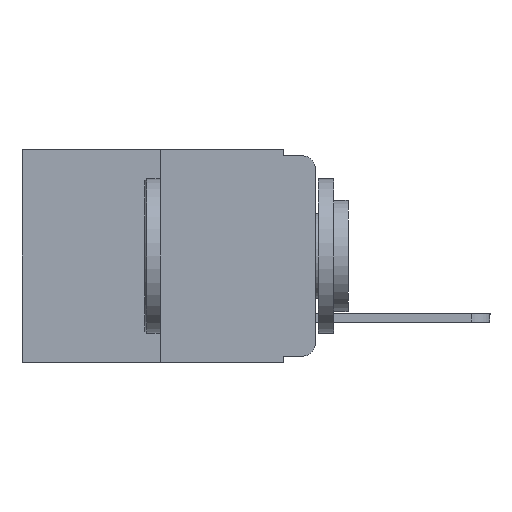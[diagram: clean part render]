
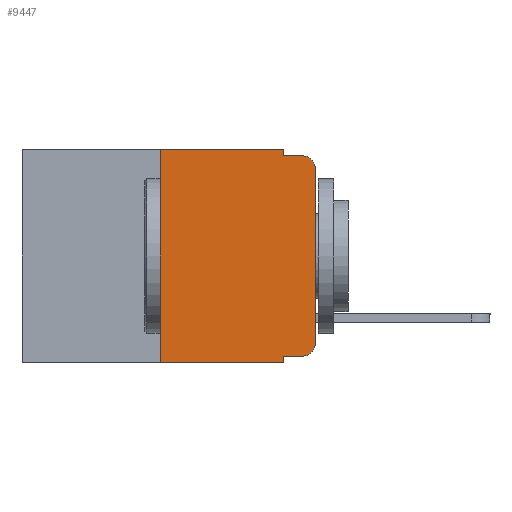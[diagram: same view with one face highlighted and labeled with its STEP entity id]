
A CAD part, left-side view. The second image highlights one B-rep face of the part: STEP entity #9447.
In plain terms, the highlighted planar face has unit normal (-1, 0, 0).
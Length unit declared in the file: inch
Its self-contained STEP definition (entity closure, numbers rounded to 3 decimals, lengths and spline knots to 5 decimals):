
#751 = EDGE_CURVE ( 'NONE', #3097, #4603, #8478, .T. ) ;
#780 = VERTEX_POINT ( 'NONE', #5957 ) ;
#983 = ORIENTED_EDGE ( 'NONE', *, *, #8936, .F. ) ;
#1001 = CARTESIAN_POINT ( 'NONE',  ( 0., 0.25, -0.343 ) ) ;
#1039 = VERTEX_POINT ( 'NONE', #2042 ) ;
#1045 = CARTESIAN_POINT ( 'NONE',  ( 0., 0.25, 0. ) ) ;
#1161 = LINE ( 'NONE', #1045, #6278 ) ;
#1274 = AXIS2_PLACEMENT_3D ( 'NONE', #11518, #5356, #2969 ) ;
#1533 = VECTOR ( 'NONE', #5927, 39.37008 ) ;
#1597 = CARTESIAN_POINT ( 'NONE',  ( 0., 0.051, 0. ) ) ;
#1614 = CARTESIAN_POINT ( 'NONE',  ( 0., 0.473, 0. ) ) ;
#1689 = ORIENTED_EDGE ( 'NONE', *, *, #6660, .F. ) ;
#1763 = CARTESIAN_POINT ( 'NONE',  ( 0., 0.02, -0.333 ) ) ;
#1821 = LINE ( 'NONE', #11740, #11657 ) ;
#1855 = LINE ( 'NONE', #9498, #1533 ) ;
#2042 = CARTESIAN_POINT ( 'NONE',  ( 0., 0.051, 0. ) ) ;
#2154 = CARTESIAN_POINT ( 'NONE',  ( 0., 0., 0. ) ) ;
#2172 = EDGE_CURVE ( 'NONE', #10506, #4603, #2993, .T. ) ;
#2265 = DIRECTION ( 'NONE',  ( 0., 0., 1. ) ) ;
#2562 = DIRECTION ( 'NONE',  ( 0., -1., 0. ) ) ;
#2915 = VECTOR ( 'NONE', #6635, 39.37008 ) ;
#2969 = DIRECTION ( 'NONE',  ( 0., 0., -1. ) ) ;
#2993 = CIRCLE ( 'NONE', #1274, 0.02 ) ;
#3045 = CARTESIAN_POINT ( 'NONE',  ( 0., 0.051, -0.01 ) ) ;
#3097 = VERTEX_POINT ( 'NONE', #11881 ) ;
#3306 = LINE ( 'NONE', #1597, #5958 ) ;
#3740 = CARTESIAN_POINT ( 'NONE',  ( 0., 0.02, -0.01 ) ) ;
#3771 = DIRECTION ( 'NONE',  ( 0., 0., -1. ) ) ;
#3786 = ORIENTED_EDGE ( 'NONE', *, *, #2172, .T. ) ;
#4203 = DIRECTION ( 'NONE',  ( 0., 0., 1. ) ) ;
#4301 = EDGE_CURVE ( 'NONE', #4403, #10506, #10620, .T. ) ;
#4403 = VERTEX_POINT ( 'NONE', #8969 ) ;
#4542 = CARTESIAN_POINT ( 'NONE',  ( 0., 0.051, -0.333 ) ) ;
#4603 = VERTEX_POINT ( 'NONE', #3740 ) ;
#5356 = DIRECTION ( 'NONE',  ( -1., 0., 0. ) ) ;
#5506 = DIRECTION ( 'NONE',  ( 0., -1., 0. ) ) ;
#5724 = PLANE ( 'NONE',  #7499 ) ;
#5766 = VECTOR ( 'NONE', #2265, 39.37008 ) ;
#5791 = ORIENTED_EDGE ( 'NONE', *, *, #4301, .T. ) ;
#5832 = EDGE_CURVE ( 'NONE', #9545, #4403, #11825, .T. ) ;
#5927 = DIRECTION ( 'NONE',  ( 0., -1., 0. ) ) ;
#5936 = EDGE_CURVE ( 'NONE', #10446, #780, #6472, .T. ) ;
#5957 = CARTESIAN_POINT ( 'NONE',  ( 0., 0.051, -0.343 ) ) ;
#5958 = VECTOR ( 'NONE', #7617, 39.37008 ) ;
#6278 = VECTOR ( 'NONE', #4203, 39.37008 ) ;
#6288 = CARTESIAN_POINT ( 'NONE',  ( 0., 0., -0.03 ) ) ;
#6472 = LINE ( 'NONE', #9164, #2915 ) ;
#6635 = DIRECTION ( 'NONE',  ( 0., -1., 0. ) ) ;
#6660 = EDGE_CURVE ( 'NONE', #10160, #1039, #1855, .T. ) ;
#7499 = AXIS2_PLACEMENT_3D ( 'NONE', #1614, #9422, #3771 ) ;
#7617 = DIRECTION ( 'NONE',  ( 0., 0., -1. ) ) ;
#7634 = CARTESIAN_POINT ( 'NONE',  ( 0., 0.051, -0.333 ) ) ;
#7655 = CARTESIAN_POINT ( 'NONE',  ( 0., 0.25, 0. ) ) ;
#7740 = EDGE_CURVE ( 'NONE', #9429, #9545, #10154, .T. ) ;
#7912 = DIRECTION ( 'NONE',  ( 0., 0., -1. ) ) ;
#8028 = EDGE_LOOP ( 'NONE', ( #5791, #3786, #8655, #11283, #1689, #983, #11489, #8999, #11919, #8332 ) ) ;
#8332 = ORIENTED_EDGE ( 'NONE', *, *, #5832, .T. ) ;
#8353 = EDGE_CURVE ( 'NONE', #9429, #780, #1821, .T. ) ;
#8392 = AXIS2_PLACEMENT_3D ( 'NONE', #8481, #8447, #7912 ) ;
#8447 = DIRECTION ( 'NONE',  ( -1., 0., 0. ) ) ;
#8448 = FACE_OUTER_BOUND ( 'NONE', #8028, .T. ) ;
#8478 = LINE ( 'NONE', #3045, #10556 ) ;
#8481 = CARTESIAN_POINT ( 'NONE',  ( 0., 0.02, -0.313 ) ) ;
#8655 = ORIENTED_EDGE ( 'NONE', *, *, #751, .F. ) ;
#8936 = EDGE_CURVE ( 'NONE', #10446, #10160, #1161, .T. ) ;
#8969 = CARTESIAN_POINT ( 'NONE',  ( 0., 0., -0.313 ) ) ;
#8999 = ORIENTED_EDGE ( 'NONE', *, *, #8353, .F. ) ;
#9164 = CARTESIAN_POINT ( 'NONE',  ( 0., 0.473, -0.343 ) ) ;
#9422 = DIRECTION ( 'NONE',  ( 1., 0., 0. ) ) ;
#9429 = VERTEX_POINT ( 'NONE', #7634 ) ;
#9447 = ADVANCED_FACE ( 'NONE', ( #8448 ), #5724, .F. ) ;
#9498 = CARTESIAN_POINT ( 'NONE',  ( 0., 0.473, 0. ) ) ;
#9545 = VERTEX_POINT ( 'NONE', #1763 ) ;
#10141 = EDGE_CURVE ( 'NONE', #1039, #3097, #3306, .T. ) ;
#10154 = LINE ( 'NONE', #4542, #12221 ) ;
#10160 = VERTEX_POINT ( 'NONE', #7655 ) ;
#10446 = VERTEX_POINT ( 'NONE', #1001 ) ;
#10506 = VERTEX_POINT ( 'NONE', #6288 ) ;
#10556 = VECTOR ( 'NONE', #2562, 39.37008 ) ;
#10620 = LINE ( 'NONE', #2154, #5766 ) ;
#11283 = ORIENTED_EDGE ( 'NONE', *, *, #10141, .F. ) ;
#11489 = ORIENTED_EDGE ( 'NONE', *, *, #5936, .T. ) ;
#11518 = CARTESIAN_POINT ( 'NONE',  ( 0., 0.02, -0.03 ) ) ;
#11657 = VECTOR ( 'NONE', #11776, 39.37008 ) ;
#11740 = CARTESIAN_POINT ( 'NONE',  ( 0., 0.051, 0. ) ) ;
#11776 = DIRECTION ( 'NONE',  ( 0., 0., -1. ) ) ;
#11825 = CIRCLE ( 'NONE', #8392, 0.02 ) ;
#11881 = CARTESIAN_POINT ( 'NONE',  ( 0., 0.051, -0.01 ) ) ;
#11919 = ORIENTED_EDGE ( 'NONE', *, *, #7740, .T. ) ;
#12221 = VECTOR ( 'NONE', #5506, 39.37008 ) ;
